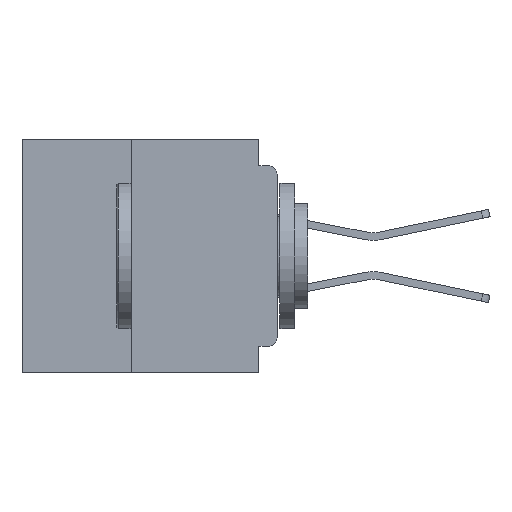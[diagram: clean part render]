
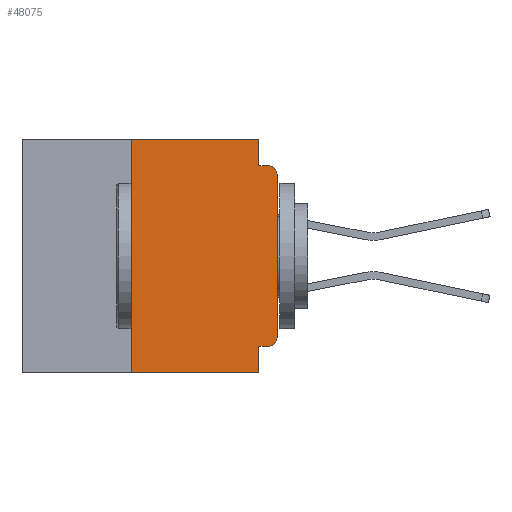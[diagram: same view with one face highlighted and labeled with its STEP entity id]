
A CAD part, left-side view. The second image highlights one B-rep face of the part: STEP entity #48075.
In plain terms, the highlighted planar face has unit normal (-1, 0, 0).
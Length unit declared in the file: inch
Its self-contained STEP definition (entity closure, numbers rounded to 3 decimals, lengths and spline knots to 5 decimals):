
#306 = CARTESIAN_POINT ( 'NONE',  ( 0., 0.437, 0. ) ) ;
#1210 = EDGE_CURVE ( 'NONE', #37337, #32942, #26025, .T. ) ;
#2801 = ORIENTED_EDGE ( 'NONE', *, *, #34965, .F. ) ;
#3977 = DIRECTION ( 'NONE',  ( 0., 0., -1. ) ) ;
#4843 = DIRECTION ( 'NONE',  ( 0., -1., 0. ) ) ;
#5195 = VERTEX_POINT ( 'NONE', #40699 ) ;
#5820 = VERTEX_POINT ( 'NONE', #9614 ) ;
#6437 = DIRECTION ( 'NONE',  ( 0., -1., 0. ) ) ;
#6745 = CARTESIAN_POINT ( 'NONE',  ( 0., 0.437, -0.4 ) ) ;
#6762 = VERTEX_POINT ( 'NONE', #31550 ) ;
#8830 = VECTOR ( 'NONE', #22859, 39.37008 ) ;
#9027 = VERTEX_POINT ( 'NONE', #53306 ) ;
#9455 = CARTESIAN_POINT ( 'NONE',  ( 0., 0.031, 0. ) ) ;
#9614 = CARTESIAN_POINT ( 'NONE',  ( 0., 0.015, -0.355 ) ) ;
#9631 = PLANE ( 'NONE',  #22420 ) ;
#10552 = DIRECTION ( 'NONE',  ( 0., 0., 1. ) ) ;
#11154 = EDGE_CURVE ( 'NONE', #5820, #53862, #30698, .T. ) ;
#12720 = CARTESIAN_POINT ( 'NONE',  ( 0., 0.25, -0.4 ) ) ;
#14187 = VECTOR ( 'NONE', #6437, 39.37008 ) ;
#14827 = CARTESIAN_POINT ( 'NONE',  ( 0., 0.25, -0.4 ) ) ;
#14995 = ORIENTED_EDGE ( 'NONE', *, *, #16662, .F. ) ;
#15826 = VECTOR ( 'NONE', #20456, 39.37008 ) ;
#16662 = EDGE_CURVE ( 'NONE', #5195, #32942, #40775, .T. ) ;
#17274 = EDGE_CURVE ( 'NONE', #5820, #5195, #51714, .T. ) ;
#18568 = DIRECTION ( 'NONE',  ( 1., 0., 0. ) ) ;
#18875 = LINE ( 'NONE', #14827, #29297 ) ;
#20218 = VERTEX_POINT ( 'NONE', #39253 ) ;
#20456 = DIRECTION ( 'NONE',  ( 0., 0., -1. ) ) ;
#20624 = LINE ( 'NONE', #9455, #8830 ) ;
#20746 = CARTESIAN_POINT ( 'NONE',  ( 0., 0.031, -0.4 ) ) ;
#20960 = DIRECTION ( 'NONE',  ( -1., 0., 0. ) ) ;
#22420 = AXIS2_PLACEMENT_3D ( 'NONE', #31759, #18568, #49505 ) ;
#22859 = DIRECTION ( 'NONE',  ( 0., 0., -1. ) ) ;
#24235 = DIRECTION ( 'NONE',  ( 0., 0., 1. ) ) ;
#26025 = LINE ( 'NONE', #6745, #14187 ) ;
#26534 = ORIENTED_EDGE ( 'NONE', *, *, #39077, .T. ) ;
#26665 = EDGE_CURVE ( 'NONE', #53862, #56256, #50741, .T. ) ;
#28111 = VECTOR ( 'NONE', #54373, 39.37008 ) ;
#28235 = VECTOR ( 'NONE', #29322, 39.37008 ) ;
#29212 = CARTESIAN_POINT ( 'NONE',  ( 0., 0.031, -0.4 ) ) ;
#29297 = VECTOR ( 'NONE', #10552, 39.37008 ) ;
#29322 = DIRECTION ( 'NONE',  ( 0., 1., 0. ) ) ;
#29495 = LINE ( 'NONE', #49942, #28111 ) ;
#30329 = EDGE_CURVE ( 'NONE', #9027, #20218, #20624, .T. ) ;
#30574 = DIRECTION ( 'NONE',  ( -1., 0., 0. ) ) ;
#30698 = CIRCLE ( 'NONE', #34138, 0.015 ) ;
#31550 = CARTESIAN_POINT ( 'NONE',  ( 0., 0.25, 0. ) ) ;
#31759 = CARTESIAN_POINT ( 'NONE',  ( 0., 0.437, 0. ) ) ;
#31771 = EDGE_CURVE ( 'NONE', #20218, #36794, #29495, .T. ) ;
#32942 = VERTEX_POINT ( 'NONE', #20746 ) ;
#33140 = CARTESIAN_POINT ( 'NONE',  ( 0., 0., 0. ) ) ;
#33799 = CARTESIAN_POINT ( 'NONE',  ( 0., 0., -0.355 ) ) ;
#34138 = AXIS2_PLACEMENT_3D ( 'NONE', #47439, #20960, #51889 ) ;
#34916 = EDGE_LOOP ( 'NONE', ( #50681, #26534, #41636, #42088, #2801, #50885, #54008, #14995, #41879, #55313 ) ) ;
#34965 = EDGE_CURVE ( 'NONE', #6762, #9027, #40024, .T. ) ;
#36794 = VERTEX_POINT ( 'NONE', #39741 ) ;
#37337 = VERTEX_POINT ( 'NONE', #12720 ) ;
#39077 = EDGE_CURVE ( 'NONE', #56256, #36794, #49761, .T. ) ;
#39253 = CARTESIAN_POINT ( 'NONE',  ( 0., 0.031, -0.045 ) ) ;
#39741 = CARTESIAN_POINT ( 'NONE',  ( 0., 0.015, -0.045 ) ) ;
#40024 = LINE ( 'NONE', #306, #51743 ) ;
#40699 = CARTESIAN_POINT ( 'NONE',  ( 0., 0.031, -0.355 ) ) ;
#40775 = LINE ( 'NONE', #29212, #15826 ) ;
#41636 = ORIENTED_EDGE ( 'NONE', *, *, #31771, .F. ) ;
#41879 = ORIENTED_EDGE ( 'NONE', *, *, #17274, .F. ) ;
#42088 = ORIENTED_EDGE ( 'NONE', *, *, #30329, .F. ) ;
#42145 = CARTESIAN_POINT ( 'NONE',  ( 0., 0., -0.06 ) ) ;
#43426 = EDGE_CURVE ( 'NONE', #37337, #6762, #18875, .T. ) ;
#47069 = CARTESIAN_POINT ( 'NONE',  ( 0., 0., -0.34 ) ) ;
#47439 = CARTESIAN_POINT ( 'NONE',  ( 0., 0.015, -0.34 ) ) ;
#47546 = FACE_OUTER_BOUND ( 'NONE', #34916, .T. ) ;
#48075 = ADVANCED_FACE ( 'NONE', ( #47546 ), #9631, .F. ) ;
#49365 = VECTOR ( 'NONE', #24235, 39.37008 ) ;
#49505 = DIRECTION ( 'NONE',  ( 0., 0., -1. ) ) ;
#49761 = CIRCLE ( 'NONE', #52865, 0.015 ) ;
#49942 = CARTESIAN_POINT ( 'NONE',  ( 0., 0., -0.045 ) ) ;
#50681 = ORIENTED_EDGE ( 'NONE', *, *, #26665, .T. ) ;
#50741 = LINE ( 'NONE', #33140, #49365 ) ;
#50885 = ORIENTED_EDGE ( 'NONE', *, *, #43426, .F. ) ;
#51714 = LINE ( 'NONE', #33799, #28235 ) ;
#51743 = VECTOR ( 'NONE', #4843, 39.37008 ) ;
#51889 = DIRECTION ( 'NONE',  ( 0., 0., -1. ) ) ;
#52865 = AXIS2_PLACEMENT_3D ( 'NONE', #57000, #30574, #3977 ) ;
#53306 = CARTESIAN_POINT ( 'NONE',  ( 0., 0.031, 0. ) ) ;
#53862 = VERTEX_POINT ( 'NONE', #47069 ) ;
#54008 = ORIENTED_EDGE ( 'NONE', *, *, #1210, .T. ) ;
#54373 = DIRECTION ( 'NONE',  ( 0., -1., 0. ) ) ;
#55313 = ORIENTED_EDGE ( 'NONE', *, *, #11154, .T. ) ;
#56256 = VERTEX_POINT ( 'NONE', #42145 ) ;
#57000 = CARTESIAN_POINT ( 'NONE',  ( 0., 0.015, -0.06 ) ) ;
